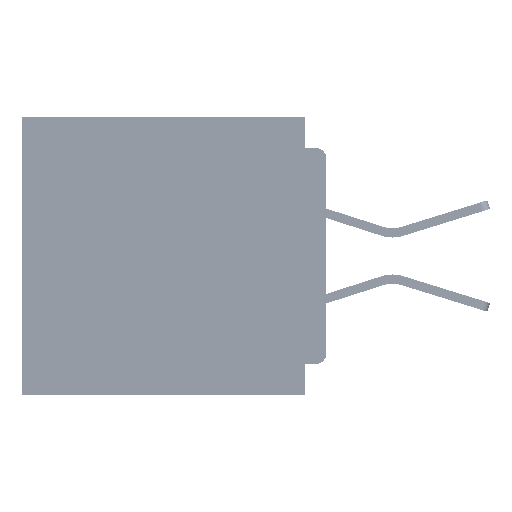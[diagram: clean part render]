
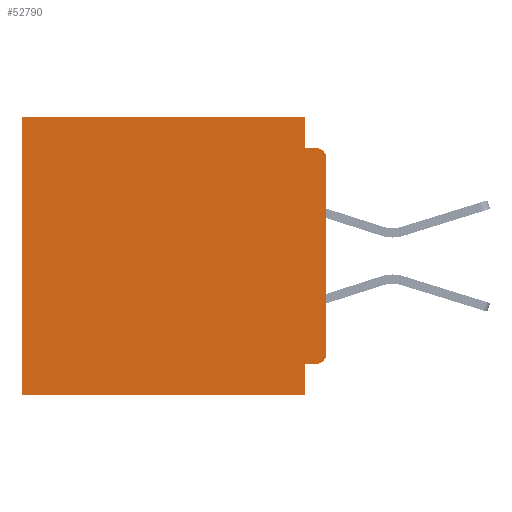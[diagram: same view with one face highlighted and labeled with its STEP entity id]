
A CAD part, left-side view. The second image highlights one B-rep face of the part: STEP entity #52790.
In plain terms, the highlighted planar face has unit normal (-1, 0, 0).
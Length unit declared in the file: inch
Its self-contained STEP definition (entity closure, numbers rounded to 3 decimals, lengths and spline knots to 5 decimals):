
#669 = VERTEX_POINT ( 'NONE', #3453 ) ;
#1283 = ORIENTED_EDGE ( 'NONE', *, *, #60965, .F. ) ;
#2574 = CARTESIAN_POINT ( 'NONE',  ( 0.3, 0.015, -0.34 ) ) ;
#2628 = EDGE_CURVE ( 'NONE', #56456, #48928, #50102, .T. ) ;
#2734 = CARTESIAN_POINT ( 'NONE',  ( 0.3, 0., -0.06 ) ) ;
#2735 = DIRECTION ( 'NONE',  ( 0., 0., -1. ) ) ;
#2812 = DIRECTION ( 'NONE',  ( -1., 0., 0. ) ) ;
#3453 = CARTESIAN_POINT ( 'NONE',  ( 0.3, 0.031, -0.355 ) ) ;
#3746 = LINE ( 'NONE', #51586, #58702 ) ;
#4239 = CARTESIAN_POINT ( 'NONE',  ( 0.3, 0.015, -0.045 ) ) ;
#4574 = LINE ( 'NONE', #43667, #31248 ) ;
#5156 = FACE_OUTER_BOUND ( 'NONE', #42181, .T. ) ;
#5651 = EDGE_CURVE ( 'NONE', #65391, #67300, #38887, .T. ) ;
#6383 = DIRECTION ( 'NONE',  ( 0., 0., -1. ) ) ;
#6661 = EDGE_CURVE ( 'NONE', #63298, #28037, #3746, .T. ) ;
#6879 = EDGE_CURVE ( 'NONE', #65391, #48928, #4574, .T. ) ;
#7283 = VECTOR ( 'NONE', #23468, 39.37008 ) ;
#8418 = LINE ( 'NONE', #28610, #20936 ) ;
#8987 = ORIENTED_EDGE ( 'NONE', *, *, #62636, .T. ) ;
#10389 = AXIS2_PLACEMENT_3D ( 'NONE', #42920, #10988, #48266 ) ;
#10988 = DIRECTION ( 'NONE',  ( 1., 0., 0. ) ) ;
#11019 = LINE ( 'NONE', #22817, #39368 ) ;
#12009 = VECTOR ( 'NONE', #31631, 39.37008 ) ;
#12046 = CARTESIAN_POINT ( 'NONE',  ( 0.3, 0.437, 0. ) ) ;
#12680 = DIRECTION ( 'NONE',  ( 0., 0., -1. ) ) ;
#17237 = ORIENTED_EDGE ( 'NONE', *, *, #51233, .F. ) ;
#17436 = DIRECTION ( 'NONE',  ( 0., 1., 0. ) ) ;
#19052 = ORIENTED_EDGE ( 'NONE', *, *, #5651, .T. ) ;
#19678 = DIRECTION ( 'NONE',  ( 0., 1., 0. ) ) ;
#20936 = VECTOR ( 'NONE', #12680, 39.37008 ) ;
#22118 = LINE ( 'NONE', #33968, #48784 ) ;
#22817 = CARTESIAN_POINT ( 'NONE',  ( 0.3, 0.437, -0.4 ) ) ;
#22843 = CARTESIAN_POINT ( 'NONE',  ( 0.3, 0., -0.355 ) ) ;
#23468 = DIRECTION ( 'NONE',  ( 0., -1., 0. ) ) ;
#24945 = VERTEX_POINT ( 'NONE', #32710 ) ;
#25149 = AXIS2_PLACEMENT_3D ( 'NONE', #31045, #68184, #36382 ) ;
#26279 = LINE ( 'NONE', #63435, #12009 ) ;
#26920 = PLANE ( 'NONE',  #10389 ) ;
#27697 = ORIENTED_EDGE ( 'NONE', *, *, #6879, .F. ) ;
#28037 = VERTEX_POINT ( 'NONE', #55207 ) ;
#28610 = CARTESIAN_POINT ( 'NONE',  ( 0.3, 0.031, 0. ) ) ;
#29987 = ORIENTED_EDGE ( 'NONE', *, *, #2628, .T. ) ;
#30651 = EDGE_CURVE ( 'NONE', #56456, #669, #66182, .T. ) ;
#31045 = CARTESIAN_POINT ( 'NONE',  ( 0.3, 0.015, -0.06 ) ) ;
#31248 = VECTOR ( 'NONE', #6383, 39.37008 ) ;
#31631 = DIRECTION ( 'NONE',  ( 0., 1., 0. ) ) ;
#32710 = CARTESIAN_POINT ( 'NONE',  ( 0.3, 0.031, 0. ) ) ;
#32729 = CARTESIAN_POINT ( 'NONE',  ( 0.3, 0.031, -0.045 ) ) ;
#33968 = CARTESIAN_POINT ( 'NONE',  ( 0.3, 0.031, -0.4 ) ) ;
#36382 = DIRECTION ( 'NONE',  ( 0., 0., -1. ) ) ;
#36808 = VERTEX_POINT ( 'NONE', #12046 ) ;
#37983 = VECTOR ( 'NONE', #17436, 39.37008 ) ;
#38887 = CIRCLE ( 'NONE', #25149, 0.015 ) ;
#39293 = CARTESIAN_POINT ( 'NONE',  ( 0.3, 0., -0.045 ) ) ;
#39337 = DIRECTION ( 'NONE',  ( 0., 0., -1. ) ) ;
#39368 = VECTOR ( 'NONE', #60014, 39.37008 ) ;
#42181 = EDGE_LOOP ( 'NONE', ( #27697, #19052, #17237, #57542, #42887, #8987, #56095, #1283, #58339, #29987 ) ) ;
#42887 = ORIENTED_EDGE ( 'NONE', *, *, #47453, .T. ) ;
#42920 = CARTESIAN_POINT ( 'NONE',  ( 0.3, 0., -0.4 ) ) ;
#43667 = CARTESIAN_POINT ( 'NONE',  ( 0.3, 0., -0.4 ) ) ;
#43869 = CARTESIAN_POINT ( 'NONE',  ( 0.3, 0.015, -0.355 ) ) ;
#47453 = EDGE_CURVE ( 'NONE', #24945, #36808, #26279, .T. ) ;
#48144 = LINE ( 'NONE', #39293, #7283 ) ;
#48266 = DIRECTION ( 'NONE',  ( 0., 0., -1. ) ) ;
#48784 = VECTOR ( 'NONE', #39337, 39.37008 ) ;
#48928 = VERTEX_POINT ( 'NONE', #55107 ) ;
#50102 = CIRCLE ( 'NONE', #56164, 0.015 ) ;
#51233 = EDGE_CURVE ( 'NONE', #51727, #67300, #48144, .T. ) ;
#51586 = CARTESIAN_POINT ( 'NONE',  ( 0.3, 0., -0.4 ) ) ;
#51727 = VERTEX_POINT ( 'NONE', #32729 ) ;
#52790 = ADVANCED_FACE ( 'NONE', ( #5156 ), #26920, .F. ) ;
#55107 = CARTESIAN_POINT ( 'NONE',  ( 0.3, 0., -0.34 ) ) ;
#55207 = CARTESIAN_POINT ( 'NONE',  ( 0.3, 0.437, -0.4 ) ) ;
#56095 = ORIENTED_EDGE ( 'NONE', *, *, #6661, .F. ) ;
#56164 = AXIS2_PLACEMENT_3D ( 'NONE', #2574, #2812, #2735 ) ;
#56456 = VERTEX_POINT ( 'NONE', #43869 ) ;
#57542 = ORIENTED_EDGE ( 'NONE', *, *, #63427, .F. ) ;
#58339 = ORIENTED_EDGE ( 'NONE', *, *, #30651, .F. ) ;
#58702 = VECTOR ( 'NONE', #19678, 39.37008 ) ;
#59267 = CARTESIAN_POINT ( 'NONE',  ( 0.3, 0.031, -0.4 ) ) ;
#60014 = DIRECTION ( 'NONE',  ( 0., 0., -1. ) ) ;
#60965 = EDGE_CURVE ( 'NONE', #669, #63298, #22118, .T. ) ;
#62636 = EDGE_CURVE ( 'NONE', #36808, #28037, #11019, .T. ) ;
#63298 = VERTEX_POINT ( 'NONE', #59267 ) ;
#63427 = EDGE_CURVE ( 'NONE', #24945, #51727, #8418, .T. ) ;
#63435 = CARTESIAN_POINT ( 'NONE',  ( 0.3, 0., 0. ) ) ;
#65391 = VERTEX_POINT ( 'NONE', #2734 ) ;
#66182 = LINE ( 'NONE', #22843, #37983 ) ;
#67300 = VERTEX_POINT ( 'NONE', #4239 ) ;
#68184 = DIRECTION ( 'NONE',  ( -1., 0., 0. ) ) ;
